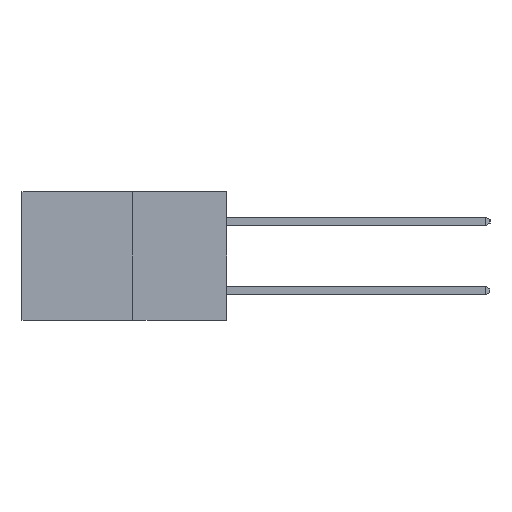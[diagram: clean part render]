
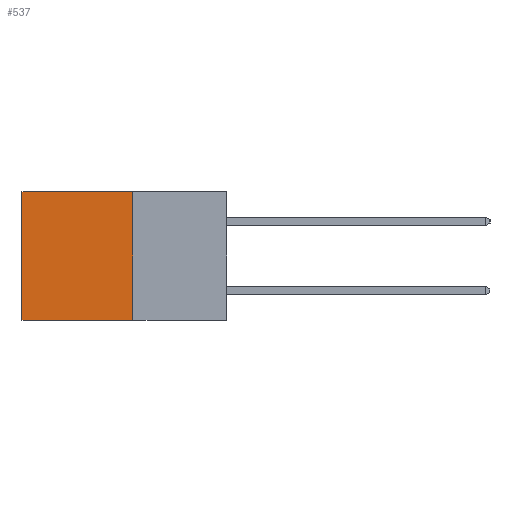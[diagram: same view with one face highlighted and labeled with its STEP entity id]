
A CAD part, left-side view. The second image highlights one B-rep face of the part: STEP entity #537.
In plain terms, the highlighted planar face has unit normal (-1, 0, 0).
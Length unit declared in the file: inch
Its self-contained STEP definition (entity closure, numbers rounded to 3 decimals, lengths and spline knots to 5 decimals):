
#455 = LINE ( 'NONE', #8219, #8757 ) ;
#537 = ADVANCED_FACE ( 'NONE', ( #6365 ), #609, .F. ) ;
#609 = PLANE ( 'NONE',  #9002 ) ;
#712 = EDGE_CURVE ( 'NONE', #5041, #7395, #5226, .T. ) ;
#774 = VERTEX_POINT ( 'NONE', #3572 ) ;
#1072 = VECTOR ( 'NONE', #4044, 39.37008 ) ;
#1190 = ORIENTED_EDGE ( 'NONE', *, *, #9861, .F. ) ;
#1201 = DIRECTION ( 'NONE',  ( 0., 0., -1. ) ) ;
#1375 = CARTESIAN_POINT ( 'NONE',  ( 0.277, 0.27, 0. ) ) ;
#1498 = VERTEX_POINT ( 'NONE', #3108 ) ;
#1926 = EDGE_LOOP ( 'NONE', ( #2141, #1190, #2731, #6914 ) ) ;
#2141 = ORIENTED_EDGE ( 'NONE', *, *, #5862, .T. ) ;
#2726 = VECTOR ( 'NONE', #3052, 39.37008 ) ;
#2731 = ORIENTED_EDGE ( 'NONE', *, *, #9185, .F. ) ;
#2851 = DIRECTION ( 'NONE',  ( 1., 0., 0. ) ) ;
#3052 = DIRECTION ( 'NONE',  ( 0., 1., 0. ) ) ;
#3108 = CARTESIAN_POINT ( 'NONE',  ( 0.277, 0.59, -0.37 ) ) ;
#3572 = CARTESIAN_POINT ( 'NONE',  ( 0.277, 0.27, -0.37 ) ) ;
#4044 = DIRECTION ( 'NONE',  ( 0., 0., -1. ) ) ;
#4221 = CARTESIAN_POINT ( 'NONE',  ( 0.277, 0.27, -0.37 ) ) ;
#4920 = CARTESIAN_POINT ( 'NONE',  ( 0.277, 0.59, -0.37 ) ) ;
#5041 = VERTEX_POINT ( 'NONE', #8834 ) ;
#5112 = LINE ( 'NONE', #4920, #1072 ) ;
#5226 = LINE ( 'NONE', #1375, #2726 ) ;
#5297 = VECTOR ( 'NONE', #7219, 39.37008 ) ;
#5544 = LINE ( 'NONE', #10291, #5297 ) ;
#5862 = EDGE_CURVE ( 'NONE', #7395, #1498, #5112, .T. ) ;
#5864 = DIRECTION ( 'NONE',  ( 0., 1., 0. ) ) ;
#6365 = FACE_OUTER_BOUND ( 'NONE', #1926, .T. ) ;
#6914 = ORIENTED_EDGE ( 'NONE', *, *, #712, .T. ) ;
#7219 = DIRECTION ( 'NONE',  ( 0., 0., -1. ) ) ;
#7395 = VERTEX_POINT ( 'NONE', #7509 ) ;
#7509 = CARTESIAN_POINT ( 'NONE',  ( 0.277, 0.59, 0. ) ) ;
#8219 = CARTESIAN_POINT ( 'NONE',  ( 0.277, 0.27, -0.37 ) ) ;
#8757 = VECTOR ( 'NONE', #5864, 39.37008 ) ;
#8834 = CARTESIAN_POINT ( 'NONE',  ( 0.277, 0.27, 0. ) ) ;
#9002 = AXIS2_PLACEMENT_3D ( 'NONE', #4221, #2851, #1201 ) ;
#9185 = EDGE_CURVE ( 'NONE', #5041, #774, #5544, .T. ) ;
#9861 = EDGE_CURVE ( 'NONE', #774, #1498, #455, .T. ) ;
#10291 = CARTESIAN_POINT ( 'NONE',  ( 0.277, 0.27, -0.37 ) ) ;
